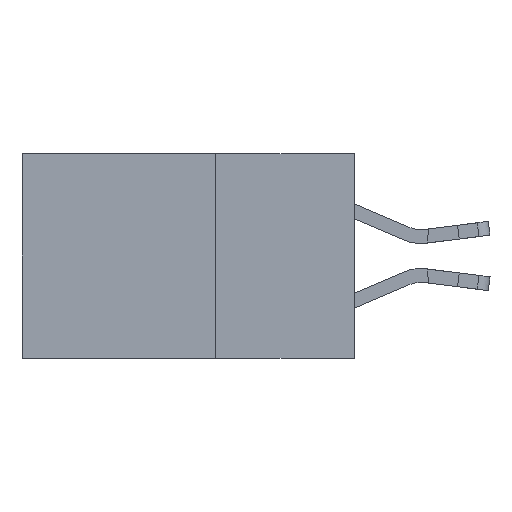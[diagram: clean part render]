
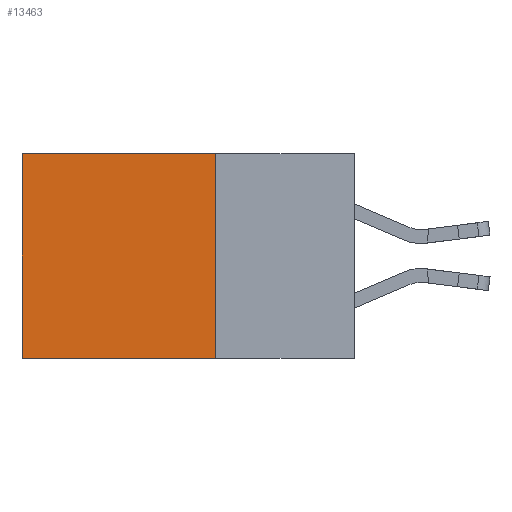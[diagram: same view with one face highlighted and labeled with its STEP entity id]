
A CAD part, left-side view. The second image highlights one B-rep face of the part: STEP entity #13463.
In plain terms, the highlighted planar face has unit normal (-1, 0, 0).
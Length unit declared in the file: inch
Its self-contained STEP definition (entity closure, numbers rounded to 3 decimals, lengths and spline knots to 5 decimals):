
#152 = EDGE_CURVE ( 'NONE', #426, #14426, #18825, .T. ) ;
#426 = VERTEX_POINT ( 'NONE', #19711 ) ;
#1062 = VERTEX_POINT ( 'NONE', #9413 ) ;
#1193 = VERTEX_POINT ( 'NONE', #15957 ) ;
#1636 = VECTOR ( 'NONE', #9540, 39.37008 ) ;
#2700 = ORIENTED_EDGE ( 'NONE', *, *, #12008, .F. ) ;
#3417 = VECTOR ( 'NONE', #15042, 39.37008 ) ;
#4160 = CARTESIAN_POINT ( 'NONE',  ( 0.298, 0.25, -0.37 ) ) ;
#4464 = CARTESIAN_POINT ( 'NONE',  ( 0.298, 0.25, 0. ) ) ;
#4552 = ORIENTED_EDGE ( 'NONE', *, *, #6506, .T. ) ;
#4663 = LINE ( 'NONE', #9423, #9024 ) ;
#5987 = EDGE_CURVE ( 'NONE', #426, #1062, #9607, .T. ) ;
#6506 = EDGE_CURVE ( 'NONE', #1062, #1193, #8975, .T. ) ;
#7282 = DIRECTION ( 'NONE',  ( 0., 1., 0. ) ) ;
#8130 = ORIENTED_EDGE ( 'NONE', *, *, #152, .F. ) ;
#8975 = LINE ( 'NONE', #19697, #3417 ) ;
#9024 = VECTOR ( 'NONE', #13779, 39.37008 ) ;
#9413 = CARTESIAN_POINT ( 'NONE',  ( 0.298, 0.6, 0. ) ) ;
#9423 = CARTESIAN_POINT ( 'NONE',  ( 0.298, 0.25, -0.37 ) ) ;
#9540 = DIRECTION ( 'NONE',  ( 0., 0., -1. ) ) ;
#9607 = LINE ( 'NONE', #4464, #17628 ) ;
#10154 = PLANE ( 'NONE',  #10822 ) ;
#10822 = AXIS2_PLACEMENT_3D ( 'NONE', #12112, #13684, #12178 ) ;
#12008 = EDGE_CURVE ( 'NONE', #14426, #1193, #4663, .T. ) ;
#12112 = CARTESIAN_POINT ( 'NONE',  ( 0.298, 0.25, 0. ) ) ;
#12178 = DIRECTION ( 'NONE',  ( 0., 0., -1. ) ) ;
#12813 = CARTESIAN_POINT ( 'NONE',  ( 0.298, 0.25, 0. ) ) ;
#13463 = ADVANCED_FACE ( 'NONE', ( #14550 ), #10154, .F. ) ;
#13684 = DIRECTION ( 'NONE',  ( 1., 0., 0. ) ) ;
#13779 = DIRECTION ( 'NONE',  ( 0., 1., 0. ) ) ;
#14426 = VERTEX_POINT ( 'NONE', #4160 ) ;
#14550 = FACE_OUTER_BOUND ( 'NONE', #16350, .T. ) ;
#15042 = DIRECTION ( 'NONE',  ( 0., 0., -1. ) ) ;
#15957 = CARTESIAN_POINT ( 'NONE',  ( 0.298, 0.6, -0.37 ) ) ;
#15982 = ORIENTED_EDGE ( 'NONE', *, *, #5987, .T. ) ;
#16350 = EDGE_LOOP ( 'NONE', ( #4552, #2700, #8130, #15982 ) ) ;
#17628 = VECTOR ( 'NONE', #7282, 39.37008 ) ;
#18825 = LINE ( 'NONE', #12813, #1636 ) ;
#19697 = CARTESIAN_POINT ( 'NONE',  ( 0.298, 0.6, 0. ) ) ;
#19711 = CARTESIAN_POINT ( 'NONE',  ( 0.298, 0.25, 0. ) ) ;
